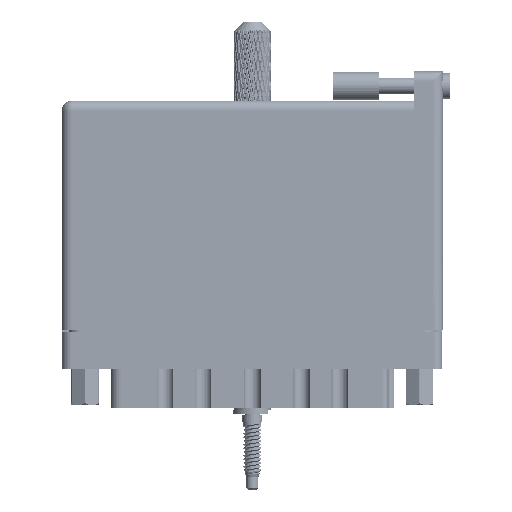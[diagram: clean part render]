
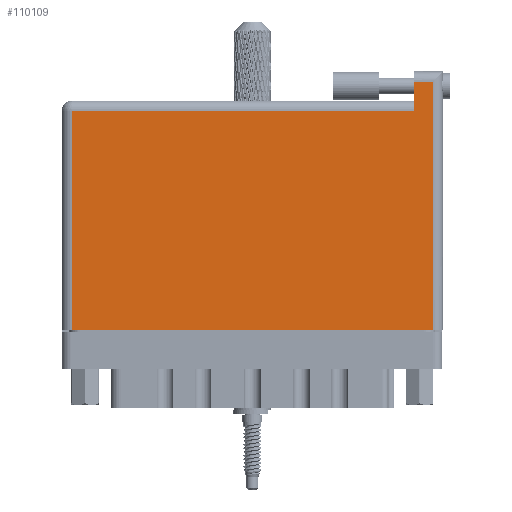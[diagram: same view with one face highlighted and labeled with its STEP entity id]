
A CAD part, front view. The second image highlights one B-rep face of the part: STEP entity #110109.
In plain terms, the highlighted face is planar.
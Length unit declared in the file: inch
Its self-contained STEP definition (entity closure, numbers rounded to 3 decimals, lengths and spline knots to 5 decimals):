
#509 = DIRECTION ( 'NONE',  ( -1., 0., 0. ) ) ;
#2245 = CARTESIAN_POINT ( 'NONE',  ( 2.403, 1.696, 0. ) ) ;
#4682 = VERTEX_POINT ( 'NONE', #72863 ) ;
#4832 = LINE ( 'NONE', #108939, #27964 ) ;
#9557 = CARTESIAN_POINT ( 'NONE',  ( 0., 1.496, 0. ) ) ;
#10895 = EDGE_CURVE ( 'NONE', #42287, #105783, #32526, .T. ) ;
#11952 = CARTESIAN_POINT ( 'NONE',  ( 2.53, 1.766, 0. ) ) ;
#14933 = LINE ( 'NONE', #9557, #123064 ) ;
#16706 = ORIENTED_EDGE ( 'NONE', *, *, #34887, .T. ) ;
#19448 = CARTESIAN_POINT ( 'NONE',  ( 0., 1.696, 0. ) ) ;
#27964 = VECTOR ( 'NONE', #99813, 39.37008 ) ;
#28112 = EDGE_CURVE ( 'NONE', #31921, #63265, #108645, .T. ) ;
#29266 = LINE ( 'NONE', #19448, #44662 ) ;
#31921 = VERTEX_POINT ( 'NONE', #93129 ) ;
#32526 = LINE ( 'NONE', #126310, #55650 ) ;
#34887 = EDGE_CURVE ( 'NONE', #63265, #63705, #48406, .T. ) ;
#38729 = ORIENTED_EDGE ( 'NONE', *, *, #10895, .T. ) ;
#42287 = VERTEX_POINT ( 'NONE', #2245 ) ;
#44662 = VECTOR ( 'NONE', #48731, 39.37008 ) ;
#45740 = EDGE_CURVE ( 'NONE', #4682, #31921, #4832, .T. ) ;
#47160 = CARTESIAN_POINT ( 'NONE',  ( 2.403, 1.496, 0. ) ) ;
#48406 = LINE ( 'NONE', #11952, #82154 ) ;
#48731 = DIRECTION ( 'NONE',  ( -1., 0., 0. ) ) ;
#50320 = CARTESIAN_POINT ( 'NONE',  ( 2.53, 0., 0. ) ) ;
#51353 = EDGE_CURVE ( 'NONE', #105783, #4682, #14933, .T. ) ;
#54137 = ORIENTED_EDGE ( 'NONE', *, *, #51353, .T. ) ;
#55650 = VECTOR ( 'NONE', #65377, 39.37008 ) ;
#63265 = VERTEX_POINT ( 'NONE', #50320 ) ;
#63705 = VERTEX_POINT ( 'NONE', #99350 ) ;
#63990 = AXIS2_PLACEMENT_3D ( 'NONE', #88289, #78814, #89172 ) ;
#65377 = DIRECTION ( 'NONE',  ( 0., -1., 0. ) ) ;
#66295 = EDGE_LOOP ( 'NONE', ( #88022, #16706, #80168, #38729, #54137, #75201 ) ) ;
#72773 = DIRECTION ( 'NONE',  ( 1., 0., 0. ) ) ;
#72863 = CARTESIAN_POINT ( 'NONE',  ( 0.07, 1.496, 0. ) ) ;
#75201 = ORIENTED_EDGE ( 'NONE', *, *, #45740, .T. ) ;
#78814 = DIRECTION ( 'NONE',  ( 0., 0., -1. ) ) ;
#80168 = ORIENTED_EDGE ( 'NONE', *, *, #107315, .T. ) ;
#82154 = VECTOR ( 'NONE', #91245, 39.37008 ) ;
#88022 = ORIENTED_EDGE ( 'NONE', *, *, #28112, .T. ) ;
#88289 = CARTESIAN_POINT ( 'NONE',  ( 0., 1.566, 0. ) ) ;
#89172 = DIRECTION ( 'NONE',  ( -1., 0., 0. ) ) ;
#91245 = DIRECTION ( 'NONE',  ( 0., 1., 0. ) ) ;
#93129 = CARTESIAN_POINT ( 'NONE',  ( 0.07, 0., 0. ) ) ;
#95169 = FACE_OUTER_BOUND ( 'NONE', #66295, .T. ) ;
#99350 = CARTESIAN_POINT ( 'NONE',  ( 2.53, 1.696, 0. ) ) ;
#99813 = DIRECTION ( 'NONE',  ( 0., -1., 0. ) ) ;
#100916 = CARTESIAN_POINT ( 'NONE',  ( 0., 0., 0. ) ) ;
#105783 = VERTEX_POINT ( 'NONE', #47160 ) ;
#107166 = VECTOR ( 'NONE', #72773, 39.37008 ) ;
#107315 = EDGE_CURVE ( 'NONE', #63705, #42287, #29266, .T. ) ;
#108268 = PLANE ( 'NONE',  #63990 ) ;
#108645 = LINE ( 'NONE', #100916, #107166 ) ;
#108939 = CARTESIAN_POINT ( 'NONE',  ( 0.07, 0., 0. ) ) ;
#110109 = ADVANCED_FACE ( 'NONE', ( #95169 ), #108268, .F. ) ;
#123064 = VECTOR ( 'NONE', #509, 39.37008 ) ;
#126310 = CARTESIAN_POINT ( 'NONE',  ( 2.403, 1.766, 0. ) ) ;
